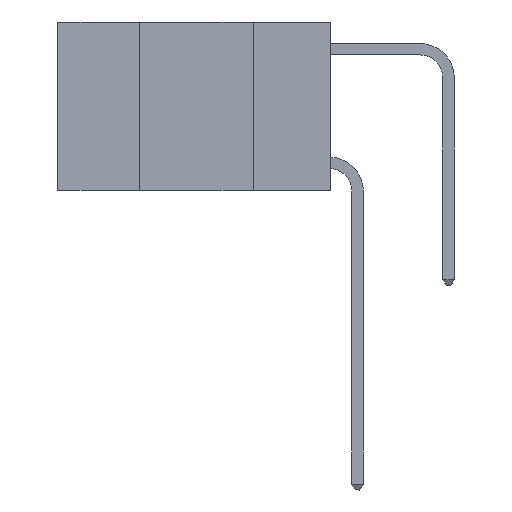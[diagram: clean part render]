
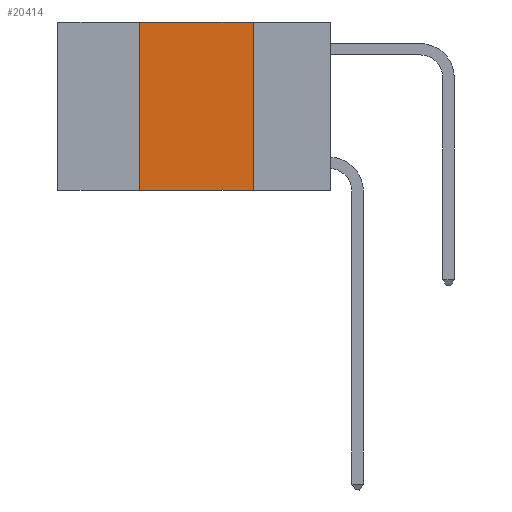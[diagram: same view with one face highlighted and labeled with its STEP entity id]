
A CAD part, left-side view. The second image highlights one B-rep face of the part: STEP entity #20414.
In plain terms, the highlighted planar face has unit normal (-1, 0, 0).
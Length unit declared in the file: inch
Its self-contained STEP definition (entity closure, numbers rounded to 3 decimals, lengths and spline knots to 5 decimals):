
#1298 = ORIENTED_EDGE ( 'NONE', *, *, #9506, .F. ) ;
#1369 = VERTEX_POINT ( 'NONE', #14450 ) ;
#1694 = CARTESIAN_POINT ( 'NONE',  ( 0., 0.42, -0.37 ) ) ;
#1802 = LINE ( 'NONE', #10242, #26299 ) ;
#2136 = PLANE ( 'NONE',  #3508 ) ;
#2317 = ORIENTED_EDGE ( 'NONE', *, *, #5546, .F. ) ;
#2509 = VECTOR ( 'NONE', #25852, 39.37008 ) ;
#2600 = CARTESIAN_POINT ( 'NONE',  ( 0., 0.17, 0. ) ) ;
#2669 = VECTOR ( 'NONE', #12201, 39.37008 ) ;
#2876 = LINE ( 'NONE', #2600, #2509 ) ;
#3508 = AXIS2_PLACEMENT_3D ( 'NONE', #18696, #23178, #10299 ) ;
#3754 = EDGE_CURVE ( 'NONE', #1369, #16303, #2876, .T. ) ;
#3773 = CARTESIAN_POINT ( 'NONE',  ( 0., 0.6, -0.37 ) ) ;
#4483 = VECTOR ( 'NONE', #26306, 39.37008 ) ;
#5546 = EDGE_CURVE ( 'NONE', #7697, #1369, #1802, .T. ) ;
#6411 = FACE_OUTER_BOUND ( 'NONE', #26979, .T. ) ;
#7697 = VERTEX_POINT ( 'NONE', #10053 ) ;
#8676 = EDGE_CURVE ( 'NONE', #23768, #16303, #22049, .T. ) ;
#9506 = EDGE_CURVE ( 'NONE', #23768, #7697, #17799, .T. ) ;
#10053 = CARTESIAN_POINT ( 'NONE',  ( 0., 0.42, 0. ) ) ;
#10067 = ORIENTED_EDGE ( 'NONE', *, *, #8676, .T. ) ;
#10242 = CARTESIAN_POINT ( 'NONE',  ( 0., 0.6, 0. ) ) ;
#10299 = DIRECTION ( 'NONE',  ( 0., 0., -1. ) ) ;
#12201 = DIRECTION ( 'NONE',  ( 0., -1., 0. ) ) ;
#14264 = DIRECTION ( 'NONE',  ( 0., -1., 0. ) ) ;
#14450 = CARTESIAN_POINT ( 'NONE',  ( 0., 0.17, 0. ) ) ;
#15764 = CARTESIAN_POINT ( 'NONE',  ( 0., 0.17, -0.37 ) ) ;
#16303 = VERTEX_POINT ( 'NONE', #15764 ) ;
#17799 = LINE ( 'NONE', #19840, #4483 ) ;
#18696 = CARTESIAN_POINT ( 'NONE',  ( 0., 0.6, 0. ) ) ;
#19840 = CARTESIAN_POINT ( 'NONE',  ( 0., 0.42, 0. ) ) ;
#20414 = ADVANCED_FACE ( 'NONE', ( #6411 ), #2136, .F. ) ;
#20643 = ORIENTED_EDGE ( 'NONE', *, *, #3754, .F. ) ;
#22049 = LINE ( 'NONE', #3773, #2669 ) ;
#23178 = DIRECTION ( 'NONE',  ( 1., 0., 0. ) ) ;
#23768 = VERTEX_POINT ( 'NONE', #1694 ) ;
#25852 = DIRECTION ( 'NONE',  ( 0., 0., -1. ) ) ;
#26299 = VECTOR ( 'NONE', #14264, 39.37008 ) ;
#26306 = DIRECTION ( 'NONE',  ( 0., 0., 1. ) ) ;
#26979 = EDGE_LOOP ( 'NONE', ( #20643, #2317, #1298, #10067 ) ) ;
